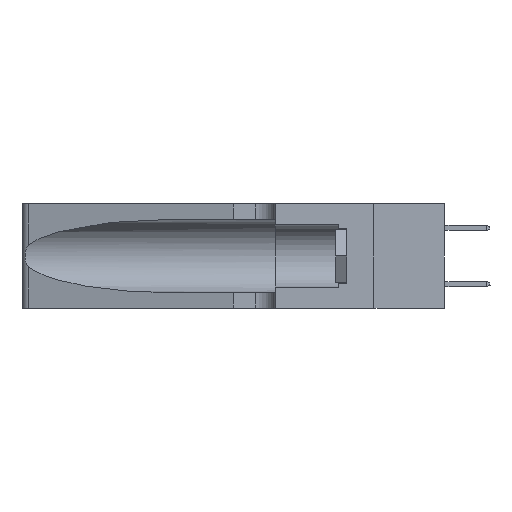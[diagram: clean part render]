
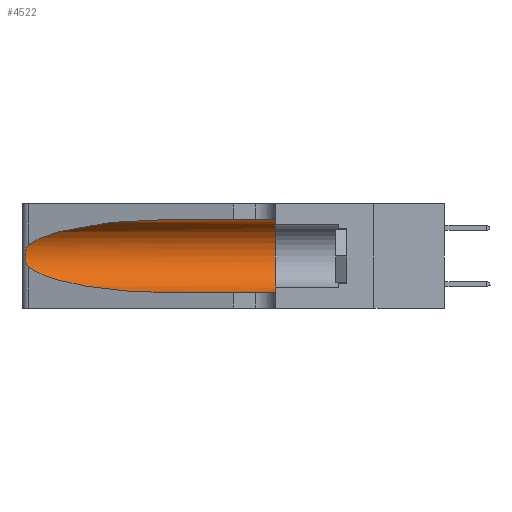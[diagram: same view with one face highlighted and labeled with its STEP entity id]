
A CAD part, left-side view. The second image highlights one B-rep face of the part: STEP entity #4522.
In plain terms, the highlighted cylindrical face has radius 3.308 mm (diameter 6.617 mm), a partial arc.
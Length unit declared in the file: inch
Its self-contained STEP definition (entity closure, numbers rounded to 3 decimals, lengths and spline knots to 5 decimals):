
#213 = LINE ( 'NONE', #11346, #30727 ) ;
#1656 = DIRECTION ( 'NONE',  ( 0., -1., 0. ) ) ;
#2009 = CARTESIAN_POINT ( 'NONE',  ( 0.25487, 1.22718, 0.14631 ) ) ;
#2877 = CARTESIAN_POINT ( 'NONE',  ( 0.2373, 1.15595, 0.08982 ) ) ;
#3294 = CARTESIAN_POINT ( 'NONE',  ( 0.25639, 1.23186, 0.15144 ) ) ;
#3544 = VERTEX_POINT ( 'NONE', #37021 ) ;
#3843 = CARTESIAN_POINT ( 'NONE',  ( 0.1305, 1.61858, 0.05475 ) ) ;
#3893 = FACE_OUTER_BOUND ( 'NONE', #43453, .T. ) ;
#4522 = ADVANCED_FACE ( 'NONE', ( #3893 ), #20551, .F. ) ;
#4648 = CARTESIAN_POINT ( 'NONE',  ( 0.2373, 1.15595, 0.28018 ) ) ;
#5809 = ORIENTED_EDGE ( 'NONE', *, *, #13593, .T. ) ;
#6442 = CARTESIAN_POINT ( 'NONE',  ( 0.1305, 0.72297, 0.05475 ) ) ;
#6875 = CARTESIAN_POINT ( 'NONE',  ( 0.25487, 1.22718, 0.14631 ) ) ;
#7433 = DIRECTION ( 'NONE',  ( 0., -1., 0. ) ) ;
#8679 = VERTEX_POINT ( 'NONE', #16393 ) ;
#9536 = CARTESIAN_POINT ( 'NONE',  ( 0.25487, 1.22718, 0.22369 ) ) ;
#10293 = CARTESIAN_POINT ( 'NONE',  ( 0.1305, 0.35, 0.05475 ) ) ;
#10322 = CARTESIAN_POINT ( 'NONE',  ( 0.25639, 1.23184, 0.21858 ) ) ;
#11346 = CARTESIAN_POINT ( 'NONE',  ( 0.1305, 1.61858, 0.31525 ) ) ;
#13593 = EDGE_CURVE ( 'NONE', #13704, #15096, #32299, .T. ) ;
#13704 = VERTEX_POINT ( 'NONE', #33491 ) ;
#13897 = CARTESIAN_POINT ( 'NONE',  ( 0.25854, 1.2359, 0.20912 ) ) ;
#15096 = VERTEX_POINT ( 'NONE', #9536 ) ;
#16365 = VERTEX_POINT ( 'NONE', #2009 ) ;
#16393 = CARTESIAN_POINT ( 'NONE',  ( 0.1305, 0.72297, 0.05475 ) ) ;
#16581 = VERTEX_POINT ( 'NONE', #10293 ) ;
#17352 = VECTOR ( 'NONE', #7433, 39.37008 ) ;
#17404 = CARTESIAN_POINT ( 'NONE',  ( 0.26075, 1.23896, 0.19203 ) ) ;
#18987 = CIRCLE ( 'NONE', #33618, 0.13025 ) ;
#19475 = ORIENTED_EDGE ( 'NONE', *, *, #23521, .T. ) ;
#20443 = ORIENTED_EDGE ( 'NONE', *, *, #30718, .F. ) ;
#20477 = EDGE_CURVE ( 'NONE', #8679, #16581, #37094, .T. ) ;
#20551 = CYLINDRICAL_SURFACE ( 'NONE', #42836, 0.13025 ) ;
#20760 = B_SPLINE_CURVE_WITH_KNOTS ( 'NONE', 3,
 ( #27889, #31442, #10322, #34919, #13897, #38417, #17404, #41906, #20983, #45401, #24512, #3294, #28043, #6875 ),
 .UNSPECIFIED., .F., .F.,
 ( 4, 2, 2, 2, 2, 2, 4 ),
 ( 0., 0.00027, 0.00053, 0.00107, 0.0016, 0.00187, 0.00214 ),
 .UNSPECIFIED. ) ;
#20789 = DIRECTION ( 'NONE',  ( 0., 1., 0. ) ) ;
#20983 = CARTESIAN_POINT ( 'NONE',  ( 0.26017, 1.23833, 0.17102 ) ) ;
#22920 = DIRECTION ( 'NONE',  ( 0., 0., -1. ) ) ;
#22939 = ORIENTED_EDGE ( 'NONE', *, *, #28920, .F. ) ;
#23521 = EDGE_CURVE ( 'NONE', #16365, #8679, #36997, .T. ) ;
#24109 = CARTESIAN_POINT ( 'NONE',  ( 0.25487, 1.22718, 0.14631 ) ) ;
#24512 = CARTESIAN_POINT ( 'NONE',  ( 0.25789, 1.23486, 0.15765 ) ) ;
#25849 = CARTESIAN_POINT ( 'NONE',  ( 0.18966, 0.96281, 0.31525 ) ) ;
#27629 = CARTESIAN_POINT ( 'NONE',  ( 0.18966, 0.96281, 0.05475 ) ) ;
#27889 = CARTESIAN_POINT ( 'NONE',  ( 0.25487, 1.22718, 0.22369 ) ) ;
#28043 = CARTESIAN_POINT ( 'NONE',  ( 0.25555, 1.22993, 0.14849 ) ) ;
#28920 = EDGE_CURVE ( 'NONE', #13704, #3544, #213, .T. ) ;
#30100 = EDGE_CURVE ( 'NONE', #15096, #16365, #20760, .T. ) ;
#30718 = EDGE_CURVE ( 'NONE', #3544, #16581, #18987, .T. ) ;
#30727 = VECTOR ( 'NONE', #35923, 39.37008 ) ;
#31442 = CARTESIAN_POINT ( 'NONE',  ( 0.25555, 1.22994, 0.2215 ) ) ;
#32299 =( BOUNDED_CURVE ( )  B_SPLINE_CURVE ( 3, ( #32897, #25849, #4648, #36382 ),
 .UNSPECIFIED., .F., .T. ) 
 B_SPLINE_CURVE_WITH_KNOTS ( ( 4, 4 ),
 ( 1.5708, 2.84003 ),
 .UNSPECIFIED. ) 
 CURVE ( )  GEOMETRIC_REPRESENTATION_ITEM ( )  RATIONAL_B_SPLINE_CURVE ( ( 1., 0.87, 0.87, 1. ) ) 
 REPRESENTATION_ITEM ( '' )  );
#32897 = CARTESIAN_POINT ( 'NONE',  ( 0.1305, 0.72297, 0.31525 ) ) ;
#33491 = CARTESIAN_POINT ( 'NONE',  ( 0.1305, 0.72297, 0.31525 ) ) ;
#33618 = AXIS2_PLACEMENT_3D ( 'NONE', #41694, #20789, #45200 ) ;
#34078 = ORIENTED_EDGE ( 'NONE', *, *, #30100, .T. ) ;
#34741 = ORIENTED_EDGE ( 'NONE', *, *, #20477, .T. ) ;
#34919 = CARTESIAN_POINT ( 'NONE',  ( 0.25787, 1.23484, 0.2124 ) ) ;
#35923 = DIRECTION ( 'NONE',  ( 0., -1., 0. ) ) ;
#36382 = CARTESIAN_POINT ( 'NONE',  ( 0.25487, 1.22718, 0.22369 ) ) ;
#36997 =( BOUNDED_CURVE ( )  B_SPLINE_CURVE ( 3, ( #24109, #2877, #27629, #6442 ),
 .UNSPECIFIED., .F., .F. ) 
 B_SPLINE_CURVE_WITH_KNOTS ( ( 4, 4 ),
 ( 3.44316, 4.71239 ),
 .UNSPECIFIED. ) 
 CURVE ( )  GEOMETRIC_REPRESENTATION_ITEM ( )  RATIONAL_B_SPLINE_CURVE ( ( 1., 0.87, 0.87, 1. ) ) 
 REPRESENTATION_ITEM ( '' )  );
#37021 = CARTESIAN_POINT ( 'NONE',  ( 0.1305, 0.35, 0.31525 ) ) ;
#37094 = LINE ( 'NONE', #3843, #17352 ) ;
#38417 = CARTESIAN_POINT ( 'NONE',  ( 0.26018, 1.23835, 0.19895 ) ) ;
#40338 = CARTESIAN_POINT ( 'NONE',  ( 0.1305, 1.61858, 0.185 ) ) ;
#41694 = CARTESIAN_POINT ( 'NONE',  ( 0.1305, 0.35, 0.185 ) ) ;
#41906 = CARTESIAN_POINT ( 'NONE',  ( 0.26075, 1.23896, 0.178 ) ) ;
#42836 = AXIS2_PLACEMENT_3D ( 'NONE', #40338, #1656, #22920 ) ;
#43453 = EDGE_LOOP ( 'NONE', ( #5809, #34078, #19475, #34741, #20443, #22939 ) ) ;
#45200 = DIRECTION ( 'NONE',  ( 0., 0., 1. ) ) ;
#45401 = CARTESIAN_POINT ( 'NONE',  ( 0.25856, 1.23593, 0.16098 ) ) ;
